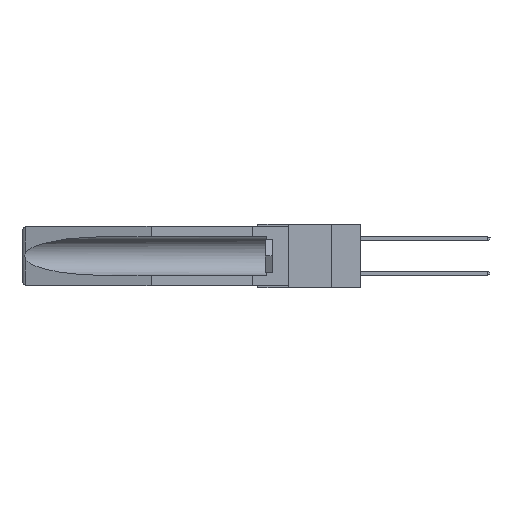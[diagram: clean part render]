
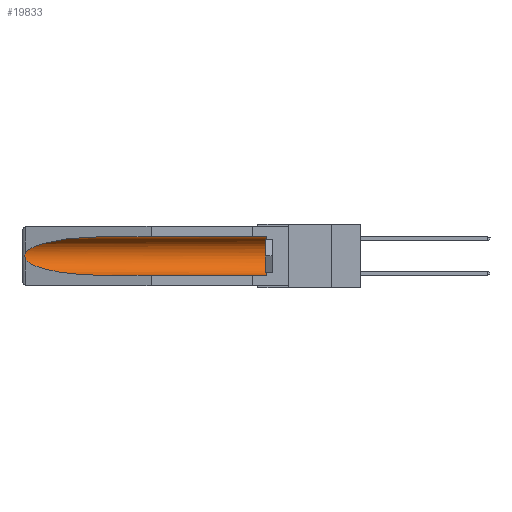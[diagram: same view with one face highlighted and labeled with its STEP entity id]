
A CAD part, left-side view. The second image highlights one B-rep face of the part: STEP entity #19833.
In plain terms, the highlighted cylindrical face has radius 2.857 mm (diameter 5.715 mm), a partial arc.
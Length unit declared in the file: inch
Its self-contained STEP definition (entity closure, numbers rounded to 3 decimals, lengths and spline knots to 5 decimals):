
#57 = CARTESIAN_POINT ( 'NONE',  ( 0.155, 1.07973, -0.284 ) ) ;
#579 = VERTEX_POINT ( 'NONE', #10894 ) ;
#651 = CARTESIAN_POINT ( 'NONE',  ( 0.155, 0.126, -0.284 ) ) ;
#778 = ORIENTED_EDGE ( 'NONE', *, *, #20960, .T. ) ;
#1027 = DIRECTION ( 'NONE',  ( 0., 1., 0. ) ) ;
#1081 = EDGE_CURVE ( 'NONE', #13035, #26062, #6802, .T. ) ;
#1337 = DIRECTION ( 'NONE',  ( 0., 1., 0. ) ) ;
#1944 = CARTESIAN_POINT ( 'NONE',  ( 0.155, -0.30754, -0.284 ) ) ;
#1948 = EDGE_CURVE ( 'NONE', #17135, #18547, #16836, .T. ) ;
#2322 = CARTESIAN_POINT ( 'NONE',  ( 0.21114, 1.30732, -0.284 ) ) ;
#2908 = CIRCLE ( 'NONE', #4900, 0.1125 ) ;
#3465 = CARTESIAN_POINT ( 'NONE',  ( 0.26655, 1.53094, -0.18657 ) ) ;
#3859 = CARTESIAN_POINT ( 'NONE',  ( 0.21114, 1.30732, -0.059 ) ) ;
#4757 = B_SPLINE_CURVE_WITH_KNOTS ( 'NONE', 3,
 ( #12283, #7730, #27741, #25435, #12190, #23305, #14521, #3465, #5672, #21188 ),
 .UNSPECIFIED., .F., .F.,
 ( 4, 2, 2, 2, 4 ),
 ( 0., 0.00029, 0.00058, 0.00087, 0.00117 ),
 .UNSPECIFIED. ) ;
#4900 = AXIS2_PLACEMENT_3D ( 'NONE', #25085, #20642, #11643 ) ;
#5672 = CARTESIAN_POINT ( 'NONE',  ( 0.26597, 1.5296, -0.19026 ) ) ;
#6170 = CARTESIAN_POINT ( 'NONE',  ( 0.155, -0.30754, -0.1715 ) ) ;
#6258 = CARTESIAN_POINT ( 'NONE',  ( 0.26537, 1.52718, -0.14972 ) ) ;
#6802 = LINE ( 'NONE', #10054, #26524 ) ;
#7730 = CARTESIAN_POINT ( 'NONE',  ( 0.26597, 1.52961, -0.15275 ) ) ;
#8218 = ORIENTED_EDGE ( 'NONE', *, *, #1081, .T. ) ;
#8829 = DIRECTION ( 'NONE',  ( 0., 1., 0. ) ) ;
#9572 = CYLINDRICAL_SURFACE ( 'NONE', #21564, 0.1125 ) ;
#9573 =( BOUNDED_CURVE ( )  B_SPLINE_CURVE ( 3, ( #14802, #3859, #17039, #6258 ),
 .UNSPECIFIED., .F., .F. ) 
 B_SPLINE_CURVE_WITH_KNOTS ( ( 4, 4 ),
 ( 4.71239, 6.08839 ),
 .UNSPECIFIED. ) 
 CURVE ( )  GEOMETRIC_REPRESENTATION_ITEM ( )  RATIONAL_B_SPLINE_CURVE ( ( 1., 0.848, 0.848, 1. ) ) 
 REPRESENTATION_ITEM ( '' )  );
#10054 = CARTESIAN_POINT ( 'NONE',  ( 0.155, -0.30754, -0.059 ) ) ;
#10226 = VECTOR ( 'NONE', #8829, 39.37008 ) ;
#10894 = CARTESIAN_POINT ( 'NONE',  ( 0.26537, 1.52718, -0.14972 ) ) ;
#11241 = CARTESIAN_POINT ( 'NONE',  ( 0.26537, 1.52718, -0.19328 ) ) ;
#11643 = DIRECTION ( 'NONE',  ( 0., 0., 1. ) ) ;
#12190 = CARTESIAN_POINT ( 'NONE',  ( 0.2675, 1.53308, -0.16763 ) ) ;
#12283 = CARTESIAN_POINT ( 'NONE',  ( 0.26537, 1.52718, -0.14972 ) ) ;
#12421 = ORIENTED_EDGE ( 'NONE', *, *, #17264, .T. ) ;
#13035 = VERTEX_POINT ( 'NONE', #22507 ) ;
#13145 = CARTESIAN_POINT ( 'NONE',  ( 0.155, 1.07973, -0.059 ) ) ;
#13686 = ORIENTED_EDGE ( 'NONE', *, *, #1948, .F. ) ;
#13700 = CARTESIAN_POINT ( 'NONE',  ( 0.155, 1.07973, -0.284 ) ) ;
#14521 = CARTESIAN_POINT ( 'NONE',  ( 0.2673, 1.53269, -0.17917 ) ) ;
#14802 = CARTESIAN_POINT ( 'NONE',  ( 0.155, 1.07973, -0.059 ) ) ;
#14812 = DIRECTION ( 'NONE',  ( 0., 0., 1. ) ) ;
#15113 = ORIENTED_EDGE ( 'NONE', *, *, #20840, .T. ) ;
#16059 = ORIENTED_EDGE ( 'NONE', *, *, #21140, .T. ) ;
#16836 = LINE ( 'NONE', #1944, #10226 ) ;
#17039 = CARTESIAN_POINT ( 'NONE',  ( 0.25451, 1.48313, -0.09465 ) ) ;
#17135 = VERTEX_POINT ( 'NONE', #651 ) ;
#17264 = EDGE_CURVE ( 'NONE', #579, #20688, #4757, .T. ) ;
#18547 = VERTEX_POINT ( 'NONE', #57 ) ;
#19833 = ADVANCED_FACE ( 'NONE', ( #28622 ), #9572, .F. ) ;
#20642 = DIRECTION ( 'NONE',  ( 0., -1., 0. ) ) ;
#20688 = VERTEX_POINT ( 'NONE', #26170 ) ;
#20840 = EDGE_CURVE ( 'NONE', #20688, #18547, #23231, .T. ) ;
#20960 = EDGE_CURVE ( 'NONE', #17135, #13035, #2908, .T. ) ;
#21140 = EDGE_CURVE ( 'NONE', #26062, #579, #9573, .T. ) ;
#21188 = CARTESIAN_POINT ( 'NONE',  ( 0.26537, 1.52718, -0.19328 ) ) ;
#21564 = AXIS2_PLACEMENT_3D ( 'NONE', #6170, #1337, #14812 ) ;
#22470 = CARTESIAN_POINT ( 'NONE',  ( 0.25451, 1.48313, -0.24835 ) ) ;
#22507 = CARTESIAN_POINT ( 'NONE',  ( 0.155, 0.126, -0.059 ) ) ;
#23231 =( BOUNDED_CURVE ( )  B_SPLINE_CURVE ( 3, ( #11241, #22470, #2322, #13700 ),
 .UNSPECIFIED., .F., .T. ) 
 B_SPLINE_CURVE_WITH_KNOTS ( ( 4, 4 ),
 ( 0.1948, 1.5708 ),
 .UNSPECIFIED. ) 
 CURVE ( )  GEOMETRIC_REPRESENTATION_ITEM ( )  RATIONAL_B_SPLINE_CURVE ( ( 1., 0.848, 0.848, 1. ) ) 
 REPRESENTATION_ITEM ( '' )  );
#23305 = CARTESIAN_POINT ( 'NONE',  ( 0.2675, 1.53308, -0.17534 ) ) ;
#25085 = CARTESIAN_POINT ( 'NONE',  ( 0.155, 0.126, -0.1715 ) ) ;
#25435 = CARTESIAN_POINT ( 'NONE',  ( 0.2673, 1.5327, -0.16383 ) ) ;
#26062 = VERTEX_POINT ( 'NONE', #13145 ) ;
#26170 = CARTESIAN_POINT ( 'NONE',  ( 0.26537, 1.52718, -0.19328 ) ) ;
#26524 = VECTOR ( 'NONE', #1027, 39.37008 ) ;
#27741 = CARTESIAN_POINT ( 'NONE',  ( 0.26654, 1.53092, -0.15636 ) ) ;
#28172 = EDGE_LOOP ( 'NONE', ( #16059, #12421, #15113, #13686, #778, #8218 ) ) ;
#28622 = FACE_OUTER_BOUND ( 'NONE', #28172, .T. ) ;
